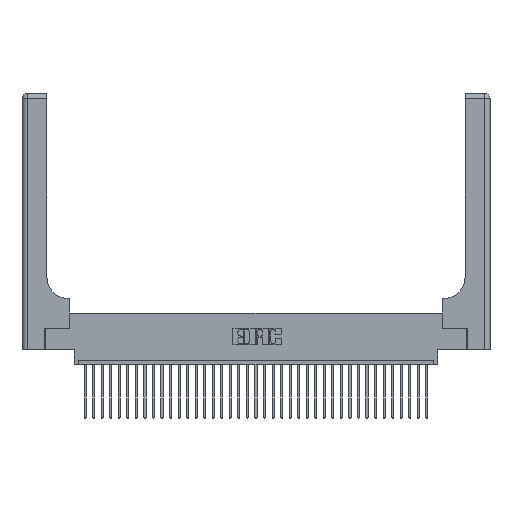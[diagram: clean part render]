
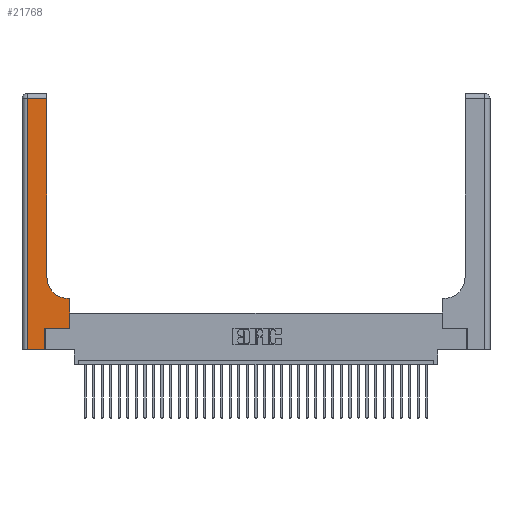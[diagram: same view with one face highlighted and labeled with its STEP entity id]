
A CAD part, top view. The second image highlights one B-rep face of the part: STEP entity #21768.
In plain terms, the highlighted planar face has unit normal (0, 0, 1).
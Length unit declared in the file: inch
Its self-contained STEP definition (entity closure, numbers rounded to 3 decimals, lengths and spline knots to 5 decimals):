
#314 = CARTESIAN_POINT ( 'NONE',  ( 0., 0., 0.37 ) ) ;
#1321 = CARTESIAN_POINT ( 'NONE',  ( 0.5415, 0.6, 0.37 ) ) ;
#2824 = VECTOR ( 'NONE', #12174, 39.37008 ) ;
#3259 = ORIENTED_EDGE ( 'NONE', *, *, #35339, .T. ) ;
#3522 = AXIS2_PLACEMENT_3D ( 'NONE', #20577, #19667, #20377 ) ;
#5134 = EDGE_CURVE ( 'NONE', #20794, #8744, #12705, .T. ) ;
#5223 = CARTESIAN_POINT ( 'NONE',  ( 0.2915, 0.85, 0.37 ) ) ;
#5771 = CARTESIAN_POINT ( 'NONE',  ( 0.06, 3., 0.37 ) ) ;
#6344 = AXIS2_PLACEMENT_3D ( 'NONE', #30189, #30313, #24661 ) ;
#6537 = CARTESIAN_POINT ( 'NONE',  ( 0.269, 0.25, 0.37 ) ) ;
#7184 = ORIENTED_EDGE ( 'NONE', *, *, #8184, .T. ) ;
#7729 = LINE ( 'NONE', #21608, #16476 ) ;
#8181 = LINE ( 'NONE', #314, #36253 ) ;
#8184 = EDGE_CURVE ( 'NONE', #30953, #20794, #15102, .T. ) ;
#8744 = VERTEX_POINT ( 'NONE', #5223 ) ;
#9194 = CARTESIAN_POINT ( 'NONE',  ( 0.269, 0., 0.37 ) ) ;
#9457 = DIRECTION ( 'NONE',  ( 1., 0., 0. ) ) ;
#9814 = VERTEX_POINT ( 'NONE', #24555 ) ;
#9999 = EDGE_CURVE ( 'NONE', #8744, #28464, #22930, .T. ) ;
#10768 = CARTESIAN_POINT ( 'NONE',  ( 0.2915, 3., 0.37 ) ) ;
#11930 = ORIENTED_EDGE ( 'NONE', *, *, #5134, .T. ) ;
#12115 = VECTOR ( 'NONE', #22482, 39.37008 ) ;
#12174 = DIRECTION ( 'NONE',  ( 0., 1., 0. ) ) ;
#12705 = CIRCLE ( 'NONE', #3522, 0.25 ) ;
#13619 = ORIENTED_EDGE ( 'NONE', *, *, #15300, .T. ) ;
#13638 = VERTEX_POINT ( 'NONE', #9194 ) ;
#13772 = CARTESIAN_POINT ( 'NONE',  ( 0.5585, 0.6, 0.37 ) ) ;
#13846 = LINE ( 'NONE', #33632, #18633 ) ;
#13972 = CARTESIAN_POINT ( 'NONE',  ( 0.2915, 2.94, 0.37 ) ) ;
#15102 = LINE ( 'NONE', #31465, #22093 ) ;
#15300 = EDGE_CURVE ( 'NONE', #9814, #19587, #16734, .T. ) ;
#16368 = CARTESIAN_POINT ( 'NONE',  ( 0.06, 0., 0.37 ) ) ;
#16476 = VECTOR ( 'NONE', #32694, 39.37008 ) ;
#16734 = LINE ( 'NONE', #6537, #21956 ) ;
#17457 = ORIENTED_EDGE ( 'NONE', *, *, #31173, .T. ) ;
#17560 = CARTESIAN_POINT ( 'NONE',  ( 0.5585, 0.25, 0.37 ) ) ;
#17639 = VECTOR ( 'NONE', #36259, 39.37008 ) ;
#18633 = VECTOR ( 'NONE', #27809, 39.37008 ) ;
#19058 = EDGE_CURVE ( 'NONE', #19292, #13638, #8181, .T. ) ;
#19187 = EDGE_CURVE ( 'NONE', #13638, #9814, #13846, .T. ) ;
#19292 = VERTEX_POINT ( 'NONE', #16368 ) ;
#19559 = LINE ( 'NONE', #5771, #12115 ) ;
#19587 = VERTEX_POINT ( 'NONE', #32977 ) ;
#19667 = DIRECTION ( 'NONE',  ( 0., 0., -1. ) ) ;
#20377 = DIRECTION ( 'NONE',  ( 1., 0., 0. ) ) ;
#20577 = CARTESIAN_POINT ( 'NONE',  ( 0.5415, 0.85, 0.37 ) ) ;
#20794 = VERTEX_POINT ( 'NONE', #1321 ) ;
#21189 = VERTEX_POINT ( 'NONE', #28908 ) ;
#21608 = CARTESIAN_POINT ( 'NONE',  ( 0., 2.94, 0.37 ) ) ;
#21768 = ADVANCED_FACE ( 'NONE', ( #24128 ), #35866, .F. ) ;
#21956 = VECTOR ( 'NONE', #9457, 39.37008 ) ;
#22093 = VECTOR ( 'NONE', #31585, 39.37008 ) ;
#22482 = DIRECTION ( 'NONE',  ( 0., -1., 0. ) ) ;
#22930 = LINE ( 'NONE', #10768, #17639 ) ;
#23469 = EDGE_LOOP ( 'NONE', ( #26460, #28309, #3259, #35300, #25358, #13619, #17457, #7184, #11930 ) ) ;
#24128 = FACE_OUTER_BOUND ( 'NONE', #23469, .T. ) ;
#24555 = CARTESIAN_POINT ( 'NONE',  ( 0.269, 0.25, 0.37 ) ) ;
#24661 = DIRECTION ( 'NONE',  ( -1., 0., 0. ) ) ;
#25152 = DIRECTION ( 'NONE',  ( 1., 0., 0. ) ) ;
#25358 = ORIENTED_EDGE ( 'NONE', *, *, #19187, .T. ) ;
#26460 = ORIENTED_EDGE ( 'NONE', *, *, #9999, .T. ) ;
#26883 = LINE ( 'NONE', #17560, #2824 ) ;
#27809 = DIRECTION ( 'NONE',  ( 0., 1., 0. ) ) ;
#28309 = ORIENTED_EDGE ( 'NONE', *, *, #35287, .T. ) ;
#28464 = VERTEX_POINT ( 'NONE', #13972 ) ;
#28908 = CARTESIAN_POINT ( 'NONE',  ( 0.06, 2.94, 0.37 ) ) ;
#30189 = CARTESIAN_POINT ( 'NONE',  ( 0., 3., 0.37 ) ) ;
#30313 = DIRECTION ( 'NONE',  ( 0., 0., -1. ) ) ;
#30953 = VERTEX_POINT ( 'NONE', #13772 ) ;
#31173 = EDGE_CURVE ( 'NONE', #19587, #30953, #26883, .T. ) ;
#31465 = CARTESIAN_POINT ( 'NONE',  ( 0.2915, 0.6, 0.37 ) ) ;
#31585 = DIRECTION ( 'NONE',  ( -1., 0., 0. ) ) ;
#32694 = DIRECTION ( 'NONE',  ( -1., 0., 0. ) ) ;
#32977 = CARTESIAN_POINT ( 'NONE',  ( 0.5585, 0.25, 0.37 ) ) ;
#33632 = CARTESIAN_POINT ( 'NONE',  ( 0.269, 0., 0.37 ) ) ;
#35287 = EDGE_CURVE ( 'NONE', #28464, #21189, #7729, .T. ) ;
#35300 = ORIENTED_EDGE ( 'NONE', *, *, #19058, .T. ) ;
#35339 = EDGE_CURVE ( 'NONE', #21189, #19292, #19559, .T. ) ;
#35866 = PLANE ( 'NONE',  #6344 ) ;
#36253 = VECTOR ( 'NONE', #25152, 39.37008 ) ;
#36259 = DIRECTION ( 'NONE',  ( 0., 1., 0. ) ) ;
